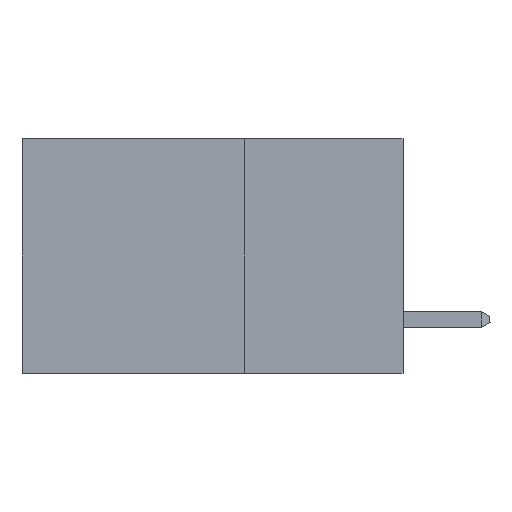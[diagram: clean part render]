
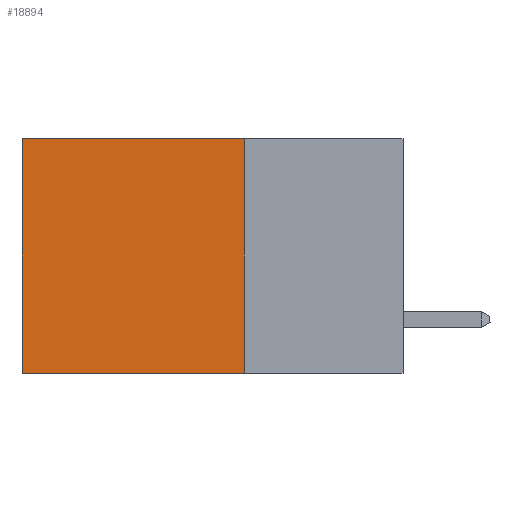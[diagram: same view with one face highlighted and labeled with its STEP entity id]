
A CAD part, left-side view. The second image highlights one B-rep face of the part: STEP entity #18894.
In plain terms, the highlighted planar face has unit normal (-1, 0, 0).
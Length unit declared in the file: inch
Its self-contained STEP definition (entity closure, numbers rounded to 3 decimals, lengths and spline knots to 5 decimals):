
#2610 = EDGE_CURVE ( 'NONE', #6273, #31803, #15516, .T. ) ;
#3443 = ORIENTED_EDGE ( 'NONE', *, *, #2610, .F. ) ;
#4475 = CARTESIAN_POINT ( 'NONE',  ( 0.2875, 0.25, -0.37 ) ) ;
#4797 = VERTEX_POINT ( 'NONE', #31540 ) ;
#6273 = VERTEX_POINT ( 'NONE', #32447 ) ;
#7746 = DIRECTION ( 'NONE',  ( 0., 1., 0. ) ) ;
#9095 = DIRECTION ( 'NONE',  ( 1., 0., 0. ) ) ;
#9555 = CARTESIAN_POINT ( 'NONE',  ( 0.2875, 0.25, 0. ) ) ;
#10477 = CARTESIAN_POINT ( 'NONE',  ( 0.2875, 0.6, 0. ) ) ;
#10517 = FACE_OUTER_BOUND ( 'NONE', #13074, .T. ) ;
#11978 = DIRECTION ( 'NONE',  ( 0., 0., -1. ) ) ;
#11983 = LINE ( 'NONE', #10477, #31829 ) ;
#12111 = EDGE_CURVE ( 'NONE', #13224, #31803, #11983, .T. ) ;
#12966 = DIRECTION ( 'NONE',  ( 0., 0., -1. ) ) ;
#13074 = EDGE_LOOP ( 'NONE', ( #13109, #3443, #31926, #36934 ) ) ;
#13109 = ORIENTED_EDGE ( 'NONE', *, *, #12111, .T. ) ;
#13112 = DIRECTION ( 'NONE',  ( 0., 0., -1. ) ) ;
#13224 = VERTEX_POINT ( 'NONE', #30905 ) ;
#13787 = DIRECTION ( 'NONE',  ( 0., 1., 0. ) ) ;
#13811 = EDGE_CURVE ( 'NONE', #4797, #13224, #21502, .T. ) ;
#14319 = EDGE_CURVE ( 'NONE', #4797, #6273, #30849, .T. ) ;
#15516 = LINE ( 'NONE', #4475, #38597 ) ;
#18894 = ADVANCED_FACE ( 'NONE', ( #10517 ), #21510, .F. ) ;
#21502 = LINE ( 'NONE', #26192, #28114 ) ;
#21510 = PLANE ( 'NONE',  #35932 ) ;
#26192 = CARTESIAN_POINT ( 'NONE',  ( 0.2875, 0.25, 0. ) ) ;
#28114 = VECTOR ( 'NONE', #7746, 39.37008 ) ;
#30849 = LINE ( 'NONE', #9555, #33679 ) ;
#30905 = CARTESIAN_POINT ( 'NONE',  ( 0.2875, 0.6, 0. ) ) ;
#31540 = CARTESIAN_POINT ( 'NONE',  ( 0.2875, 0.25, 0. ) ) ;
#31803 = VERTEX_POINT ( 'NONE', #32975 ) ;
#31829 = VECTOR ( 'NONE', #13112, 39.37008 ) ;
#31926 = ORIENTED_EDGE ( 'NONE', *, *, #14319, .F. ) ;
#32447 = CARTESIAN_POINT ( 'NONE',  ( 0.2875, 0.25, -0.37 ) ) ;
#32975 = CARTESIAN_POINT ( 'NONE',  ( 0.2875, 0.6, -0.37 ) ) ;
#33215 = CARTESIAN_POINT ( 'NONE',  ( 0.2875, 0.25, 0. ) ) ;
#33679 = VECTOR ( 'NONE', #12966, 39.37008 ) ;
#35932 = AXIS2_PLACEMENT_3D ( 'NONE', #33215, #9095, #11978 ) ;
#36934 = ORIENTED_EDGE ( 'NONE', *, *, #13811, .T. ) ;
#38597 = VECTOR ( 'NONE', #13787, 39.37008 ) ;
